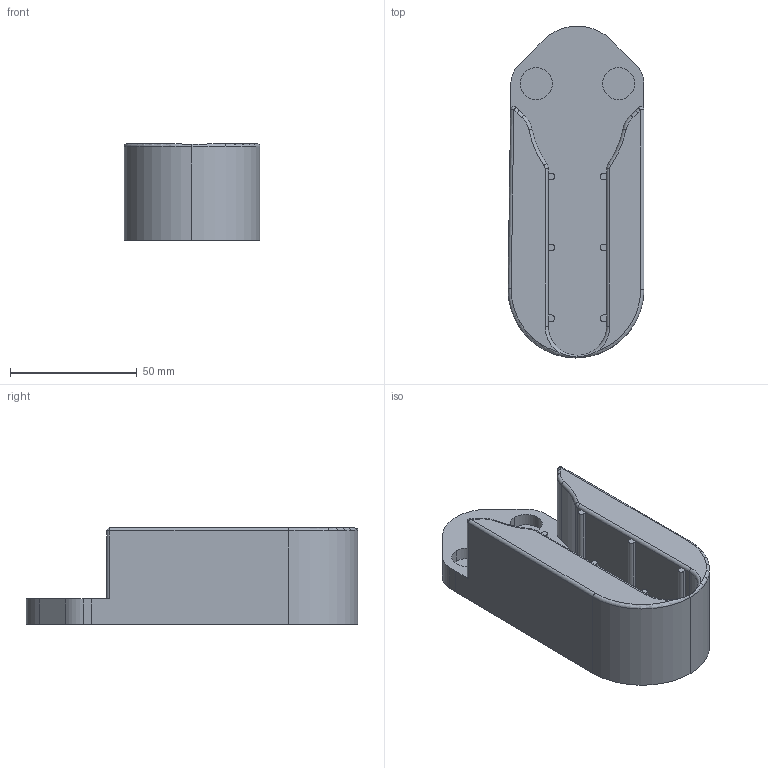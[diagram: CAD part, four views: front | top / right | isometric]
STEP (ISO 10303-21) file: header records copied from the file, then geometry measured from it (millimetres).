
FILE_DESCRIPTION (( 'STEP AP214' ), '1' );
FILE_NAME ('Butt Cover.STEP', '2013-12-11T22:25:40', ( 'elpi' ), ( '' ), 'SwSTEP 2.0', 'SolidWorks 2013', '' );
FILE_SCHEMA (( 'AUTOMOTIVE_DESIGN' ));
Length unit declared in the file: inch
Products named in the file (1): Butt Cover
Bounding box: 53.66 x 130.98 x 38.1 mm (x, y, z)
Volume: 129846.1 mm3; surface area: 29955.9 mm2
Topology: 1 solids, 1 shells, 101 faces, 249 edges, 154 vertices
Faces by surface type: cylinder 44, plane 43, torus 12, sphere 2
Entity records: 3010 total; most frequent: DIRECTION 552, CARTESIAN_POINT 523, ORIENTED_EDGE 490, EDGE_CURVE 245, AXIS2_PLACEMENT_3D 209, VERTEX_POINT 152, LINE 134, VECTOR 134
